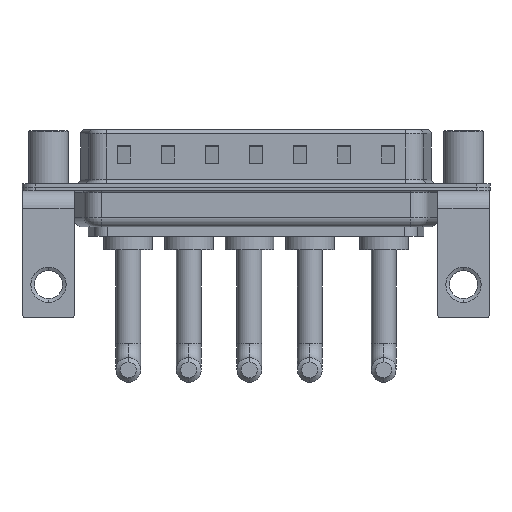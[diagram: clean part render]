
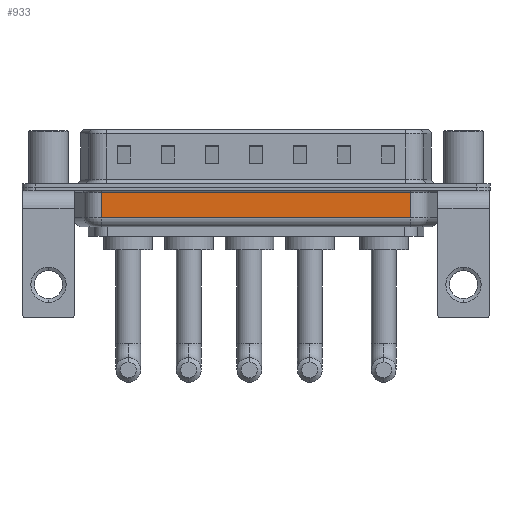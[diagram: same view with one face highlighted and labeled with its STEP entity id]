
A CAD part, front view. The second image highlights one B-rep face of the part: STEP entity #933.
In plain terms, the highlighted planar face has unit normal (0, -1, 0).
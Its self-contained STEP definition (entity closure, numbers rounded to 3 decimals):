
#583 = EDGE_LOOP ( 'NONE', ( #11651, #16353, #6860, #2072 ) ) ;
#689 = CARTESIAN_POINT ( 'NONE',  ( 41.044, -5.35, -0.65 ) ) ;
#746 = VERTEX_POINT ( 'NONE', #12851 ) ;
#865 = CARTESIAN_POINT ( 'NONE',  ( 6.006, -5.35, -3.5 ) ) ;
#933 = ADVANCED_FACE ( 'NONE', ( #1453 ), #11972, .F. ) ;
#1453 = FACE_OUTER_BOUND ( 'NONE', #583, .T. ) ;
#1514 = DIRECTION ( 'NONE',  ( 0., 0., 1. ) ) ;
#1851 = CARTESIAN_POINT ( 'NONE',  ( 6.006, -5.35, -4.5 ) ) ;
#1939 = LINE ( 'NONE', #14942, #11479 ) ;
#2072 = ORIENTED_EDGE ( 'NONE', *, *, #12597, .T. ) ;
#2818 = LINE ( 'NONE', #3861, #11114 ) ;
#3131 = EDGE_CURVE ( 'NONE', #9615, #13966, #9985, .T. ) ;
#3723 = EDGE_CURVE ( 'NONE', #9615, #746, #15802, .T. ) ;
#3861 = CARTESIAN_POINT ( 'NONE',  ( 6.006, -5.35, -0.65 ) ) ;
#5774 = CARTESIAN_POINT ( 'NONE',  ( 6.006, -5.35, -3.5 ) ) ;
#6860 = ORIENTED_EDGE ( 'NONE', *, *, #16186, .T. ) ;
#7148 = DIRECTION ( 'NONE',  ( 0., 0., 1. ) ) ;
#8022 = DIRECTION ( 'NONE',  ( -1., 0., 0. ) ) ;
#8264 = VECTOR ( 'NONE', #11112, 1000. ) ;
#9107 = VECTOR ( 'NONE', #1514, 1000. ) ;
#9615 = VERTEX_POINT ( 'NONE', #5774 ) ;
#9985 = LINE ( 'NONE', #865, #8264 ) ;
#10664 = CARTESIAN_POINT ( 'NONE',  ( 6.006, -5.35, -4.5 ) ) ;
#11088 = DIRECTION ( 'NONE',  ( 0., 1., 0. ) ) ;
#11112 = DIRECTION ( 'NONE',  ( 1., 0., 0. ) ) ;
#11114 = VECTOR ( 'NONE', #8022, 1000. ) ;
#11231 = AXIS2_PLACEMENT_3D ( 'NONE', #1851, #11088, #12299 ) ;
#11479 = VECTOR ( 'NONE', #7148, 1000. ) ;
#11549 = CARTESIAN_POINT ( 'NONE',  ( 41.044, -5.35, -3.5 ) ) ;
#11651 = ORIENTED_EDGE ( 'NONE', *, *, #3723, .F. ) ;
#11972 = PLANE ( 'NONE',  #11231 ) ;
#12299 = DIRECTION ( 'NONE',  ( 0., 0., 1. ) ) ;
#12597 = EDGE_CURVE ( 'NONE', #14235, #746, #2818, .T. ) ;
#12851 = CARTESIAN_POINT ( 'NONE',  ( 6.006, -5.35, -0.65 ) ) ;
#13966 = VERTEX_POINT ( 'NONE', #11549 ) ;
#14235 = VERTEX_POINT ( 'NONE', #689 ) ;
#14942 = CARTESIAN_POINT ( 'NONE',  ( 41.044, -5.35, -4.5 ) ) ;
#15802 = LINE ( 'NONE', #10664, #9107 ) ;
#16186 = EDGE_CURVE ( 'NONE', #13966, #14235, #1939, .T. ) ;
#16353 = ORIENTED_EDGE ( 'NONE', *, *, #3131, .T. ) ;
